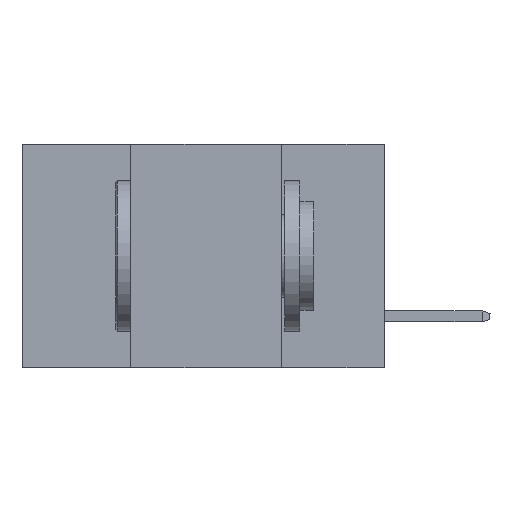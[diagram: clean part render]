
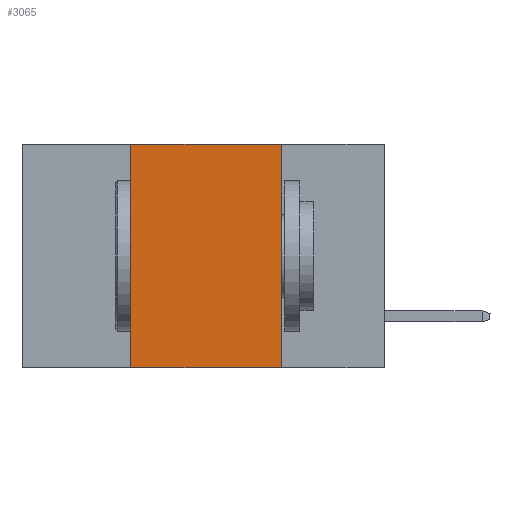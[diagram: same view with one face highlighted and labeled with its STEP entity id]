
A CAD part, left-side view. The second image highlights one B-rep face of the part: STEP entity #3065.
In plain terms, the highlighted planar face has unit normal (-1, 0, 0).
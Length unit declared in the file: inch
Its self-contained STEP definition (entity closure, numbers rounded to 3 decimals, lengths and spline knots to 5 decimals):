
#463 = DIRECTION ( 'NONE',  ( 0., -1., 0. ) ) ;
#1606 = VECTOR ( 'NONE', #3547, 39.37008 ) ;
#1854 = CARTESIAN_POINT ( 'NONE',  ( 0., 0.42, -0.37 ) ) ;
#2181 = ORIENTED_EDGE ( 'NONE', *, *, #8058, .F. ) ;
#2333 = ORIENTED_EDGE ( 'NONE', *, *, #7391, .T. ) ;
#2490 = CARTESIAN_POINT ( 'NONE',  ( 0., 0.17, -0.37 ) ) ;
#2828 = ORIENTED_EDGE ( 'NONE', *, *, #9246, .F. ) ;
#2872 = EDGE_LOOP ( 'NONE', ( #12200, #2828, #2181, #2333 ) ) ;
#2905 = VECTOR ( 'NONE', #10244, 39.37008 ) ;
#3065 = ADVANCED_FACE ( 'NONE', ( #5737 ), #9534, .F. ) ;
#3140 = EDGE_CURVE ( 'NONE', #9043, #4348, #10588, .T. ) ;
#3378 = VERTEX_POINT ( 'NONE', #9060 ) ;
#3547 = DIRECTION ( 'NONE',  ( 0., 0., -1. ) ) ;
#3714 = DIRECTION ( 'NONE',  ( 0., 0., 1. ) ) ;
#4348 = VERTEX_POINT ( 'NONE', #5275 ) ;
#4399 = VECTOR ( 'NONE', #3714, 39.37008 ) ;
#4648 = LINE ( 'NONE', #7682, #4399 ) ;
#5015 = LINE ( 'NONE', #5213, #2905 ) ;
#5213 = CARTESIAN_POINT ( 'NONE',  ( 0., 0.6, -0.37 ) ) ;
#5275 = CARTESIAN_POINT ( 'NONE',  ( 0., 0.17, -0.37 ) ) ;
#5533 = DIRECTION ( 'NONE',  ( 1., 0., 0. ) ) ;
#5737 = FACE_OUTER_BOUND ( 'NONE', #2872, .T. ) ;
#5931 = CARTESIAN_POINT ( 'NONE',  ( 0., 0.17, 0. ) ) ;
#6287 = AXIS2_PLACEMENT_3D ( 'NONE', #6597, #5533, #9738 ) ;
#6597 = CARTESIAN_POINT ( 'NONE',  ( 0., 0.6, 0. ) ) ;
#7391 = EDGE_CURVE ( 'NONE', #11123, #4348, #5015, .T. ) ;
#7682 = CARTESIAN_POINT ( 'NONE',  ( 0., 0.42, -0.37 ) ) ;
#8058 = EDGE_CURVE ( 'NONE', #11123, #3378, #4648, .T. ) ;
#9043 = VERTEX_POINT ( 'NONE', #5931 ) ;
#9060 = CARTESIAN_POINT ( 'NONE',  ( 0., 0.42, 0. ) ) ;
#9246 = EDGE_CURVE ( 'NONE', #3378, #9043, #9453, .T. ) ;
#9453 = LINE ( 'NONE', #10383, #11986 ) ;
#9534 = PLANE ( 'NONE',  #6287 ) ;
#9738 = DIRECTION ( 'NONE',  ( 0., 0., -1. ) ) ;
#10244 = DIRECTION ( 'NONE',  ( 0., -1., 0. ) ) ;
#10383 = CARTESIAN_POINT ( 'NONE',  ( 0., 0.6, 0. ) ) ;
#10588 = LINE ( 'NONE', #2490, #1606 ) ;
#11123 = VERTEX_POINT ( 'NONE', #1854 ) ;
#11986 = VECTOR ( 'NONE', #463, 39.37008 ) ;
#12200 = ORIENTED_EDGE ( 'NONE', *, *, #3140, .F. ) ;
